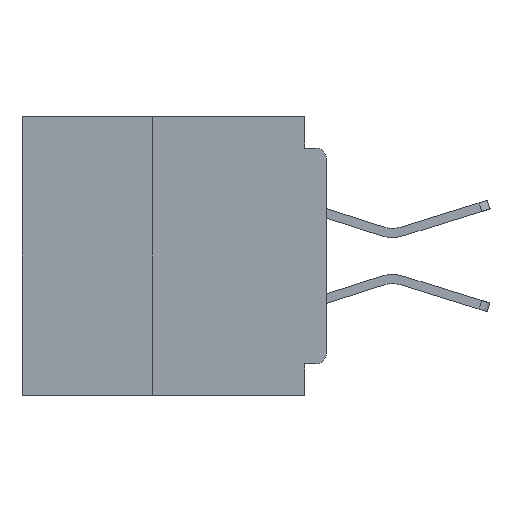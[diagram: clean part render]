
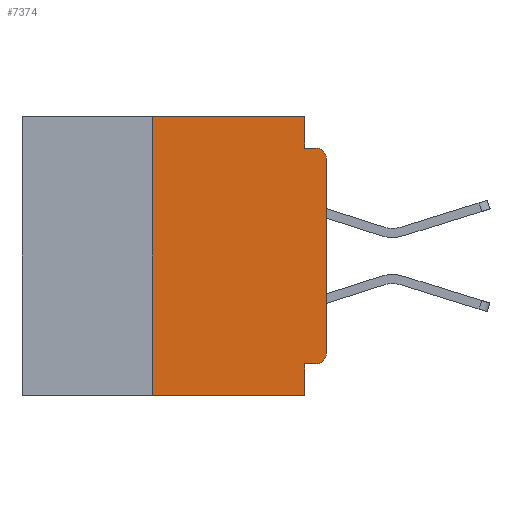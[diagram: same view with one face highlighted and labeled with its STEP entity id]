
A CAD part, left-side view. The second image highlights one B-rep face of the part: STEP entity #7374.
In plain terms, the highlighted planar face has unit normal (-1, 0, 0).
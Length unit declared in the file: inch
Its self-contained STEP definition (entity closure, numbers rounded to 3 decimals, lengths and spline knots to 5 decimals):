
#557 = CARTESIAN_POINT ( 'NONE',  ( 0., 0., -0.34 ) ) ;
#926 = DIRECTION ( 'NONE',  ( 0., 0., -1. ) ) ;
#2706 = CIRCLE ( 'NONE', #50737, 0.015 ) ;
#5500 = DIRECTION ( 'NONE',  ( 0., -1., 0. ) ) ;
#6102 = VERTEX_POINT ( 'NONE', #10890 ) ;
#7367 = EDGE_CURVE ( 'NONE', #14678, #29654, #45673, .T. ) ;
#7374 = ADVANCED_FACE ( 'NONE', ( #57454 ), #56426, .F. ) ;
#7532 = LINE ( 'NONE', #64428, #46319 ) ;
#10446 = LINE ( 'NONE', #25915, #46039 ) ;
#10539 = DIRECTION ( 'NONE',  ( 0., 0., 1. ) ) ;
#10890 = CARTESIAN_POINT ( 'NONE',  ( 0., 0.25, -0.4 ) ) ;
#10951 = DIRECTION ( 'NONE',  ( 0., -1., 0. ) ) ;
#14678 = VERTEX_POINT ( 'NONE', #29207 ) ;
#15130 = AXIS2_PLACEMENT_3D ( 'NONE', #26006, #31317, #926 ) ;
#15814 = CARTESIAN_POINT ( 'NONE',  ( 0., 0.437, 0. ) ) ;
#16139 = ORIENTED_EDGE ( 'NONE', *, *, #24276, .T. ) ;
#16507 = VERTEX_POINT ( 'NONE', #23013 ) ;
#17527 = ORIENTED_EDGE ( 'NONE', *, *, #58796, .T. ) ;
#17802 = EDGE_CURVE ( 'NONE', #27163, #48266, #2706, .T. ) ;
#18357 = CARTESIAN_POINT ( 'NONE',  ( 0., 0.031, -0.4 ) ) ;
#18399 = ORIENTED_EDGE ( 'NONE', *, *, #30878, .F. ) ;
#18442 = CARTESIAN_POINT ( 'NONE',  ( 0., 0.015, -0.045 ) ) ;
#18717 = ORIENTED_EDGE ( 'NONE', *, *, #26057, .F. ) ;
#19325 = AXIS2_PLACEMENT_3D ( 'NONE', #29721, #64869, #34830 ) ;
#19854 = CARTESIAN_POINT ( 'NONE',  ( 0., 0.437, -0.4 ) ) ;
#21145 = ORIENTED_EDGE ( 'NONE', *, *, #7367, .F. ) ;
#21634 = ORIENTED_EDGE ( 'NONE', *, *, #44553, .F. ) ;
#22022 = ORIENTED_EDGE ( 'NONE', *, *, #51494, .T. ) ;
#22503 = VECTOR ( 'NONE', #5500, 39.37008 ) ;
#23013 = CARTESIAN_POINT ( 'NONE',  ( 0., 0.031, -0.355 ) ) ;
#23099 = LINE ( 'NONE', #30681, #35000 ) ;
#23995 = ORIENTED_EDGE ( 'NONE', *, *, #54179, .F. ) ;
#24276 = EDGE_CURVE ( 'NONE', #48266, #60035, #23099, .T. ) ;
#24356 = DIRECTION ( 'NONE',  ( 0., 1., 0. ) ) ;
#24644 = ORIENTED_EDGE ( 'NONE', *, *, #26362, .F. ) ;
#25497 = CIRCLE ( 'NONE', #19325, 0.015 ) ;
#25660 = CARTESIAN_POINT ( 'NONE',  ( 0., 0., -0.045 ) ) ;
#25915 = CARTESIAN_POINT ( 'NONE',  ( 0., 0.031, 0. ) ) ;
#26006 = CARTESIAN_POINT ( 'NONE',  ( 0., 0.437, 0. ) ) ;
#26057 = EDGE_CURVE ( 'NONE', #29654, #36234, #10446, .T. ) ;
#26177 = CARTESIAN_POINT ( 'NONE',  ( 0., 0.031, -0.045 ) ) ;
#26191 = VECTOR ( 'NONE', #29638, 39.37008 ) ;
#26362 = EDGE_CURVE ( 'NONE', #27163, #16507, #53860, .T. ) ;
#26716 = ORIENTED_EDGE ( 'NONE', *, *, #17802, .T. ) ;
#27163 = VERTEX_POINT ( 'NONE', #46345 ) ;
#27777 = LINE ( 'NONE', #54781, #26191 ) ;
#28055 = VERTEX_POINT ( 'NONE', #18357 ) ;
#28158 = LINE ( 'NONE', #19854, #40075 ) ;
#28542 = DIRECTION ( 'NONE',  ( -1., 0., 0. ) ) ;
#29207 = CARTESIAN_POINT ( 'NONE',  ( 0., 0.25, 0. ) ) ;
#29260 = DIRECTION ( 'NONE',  ( 0., 0., 1. ) ) ;
#29638 = DIRECTION ( 'NONE',  ( 0., 0., -1. ) ) ;
#29654 = VERTEX_POINT ( 'NONE', #41534 ) ;
#29721 = CARTESIAN_POINT ( 'NONE',  ( 0., 0.015, -0.06 ) ) ;
#30681 = CARTESIAN_POINT ( 'NONE',  ( 0., 0., 0. ) ) ;
#30878 = EDGE_CURVE ( 'NONE', #36234, #58658, #35999, .T. ) ;
#31317 = DIRECTION ( 'NONE',  ( 1., 0., 0. ) ) ;
#32229 = VECTOR ( 'NONE', #10951, 39.37008 ) ;
#34830 = DIRECTION ( 'NONE',  ( 0., 0., -1. ) ) ;
#35000 = VECTOR ( 'NONE', #10539, 39.37008 ) ;
#35999 = LINE ( 'NONE', #25660, #22503 ) ;
#36110 = DIRECTION ( 'NONE',  ( 0., 0., -1. ) ) ;
#36234 = VERTEX_POINT ( 'NONE', #26177 ) ;
#39626 = CARTESIAN_POINT ( 'NONE',  ( 0., 0., -0.355 ) ) ;
#40075 = VECTOR ( 'NONE', #55175, 39.37008 ) ;
#41534 = CARTESIAN_POINT ( 'NONE',  ( 0., 0.031, 0. ) ) ;
#43955 = CARTESIAN_POINT ( 'NONE',  ( 0., 0., -0.06 ) ) ;
#44553 = EDGE_CURVE ( 'NONE', #6102, #14678, #7532, .T. ) ;
#45659 = EDGE_LOOP ( 'NONE', ( #16139, #17527, #18399, #18717, #21145, #21634, #22022, #23995, #24644, #26716 ) ) ;
#45673 = LINE ( 'NONE', #15814, #32229 ) ;
#46039 = VECTOR ( 'NONE', #36110, 39.37008 ) ;
#46319 = VECTOR ( 'NONE', #29260, 39.37008 ) ;
#46345 = CARTESIAN_POINT ( 'NONE',  ( 0., 0.015, -0.355 ) ) ;
#48266 = VERTEX_POINT ( 'NONE', #557 ) ;
#50737 = AXIS2_PLACEMENT_3D ( 'NONE', #58718, #28542, #63728 ) ;
#51494 = EDGE_CURVE ( 'NONE', #6102, #28055, #28158, .T. ) ;
#52284 = VECTOR ( 'NONE', #24356, 39.37008 ) ;
#53860 = LINE ( 'NONE', #39626, #52284 ) ;
#54179 = EDGE_CURVE ( 'NONE', #16507, #28055, #27777, .T. ) ;
#54781 = CARTESIAN_POINT ( 'NONE',  ( 0., 0.031, -0.4 ) ) ;
#55175 = DIRECTION ( 'NONE',  ( 0., -1., 0. ) ) ;
#56426 = PLANE ( 'NONE',  #15130 ) ;
#57454 = FACE_OUTER_BOUND ( 'NONE', #45659, .T. ) ;
#58658 = VERTEX_POINT ( 'NONE', #18442 ) ;
#58718 = CARTESIAN_POINT ( 'NONE',  ( 0., 0.015, -0.34 ) ) ;
#58796 = EDGE_CURVE ( 'NONE', #60035, #58658, #25497, .T. ) ;
#60035 = VERTEX_POINT ( 'NONE', #43955 ) ;
#63728 = DIRECTION ( 'NONE',  ( 0., 0., -1. ) ) ;
#64428 = CARTESIAN_POINT ( 'NONE',  ( 0., 0.25, -0.4 ) ) ;
#64869 = DIRECTION ( 'NONE',  ( -1., 0., 0. ) ) ;
